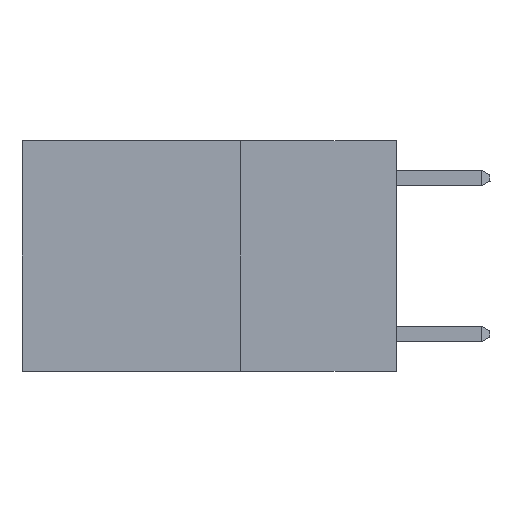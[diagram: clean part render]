
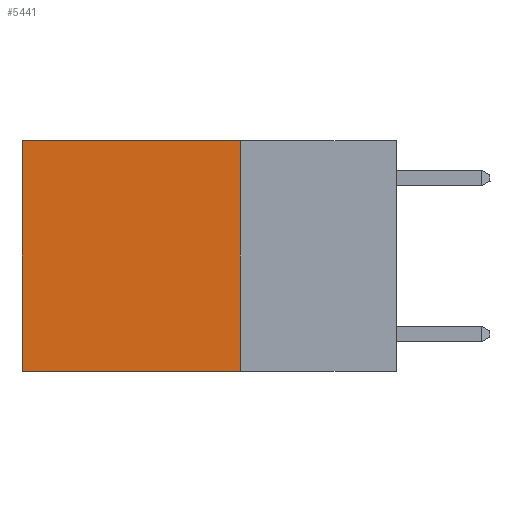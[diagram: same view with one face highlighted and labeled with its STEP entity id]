
A CAD part, left-side view. The second image highlights one B-rep face of the part: STEP entity #5441.
In plain terms, the highlighted planar face has unit normal (-1, 0, 0).
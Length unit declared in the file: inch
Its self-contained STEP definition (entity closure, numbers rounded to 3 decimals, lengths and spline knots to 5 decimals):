
#237 = CARTESIAN_POINT ( 'NONE',  ( 0.2625, 0.25, -0.37 ) ) ;
#318 = ORIENTED_EDGE ( 'NONE', *, *, #1720, .T. ) ;
#560 = ORIENTED_EDGE ( 'NONE', *, *, #9126, .T. ) ;
#706 = ORIENTED_EDGE ( 'NONE', *, *, #6501, .F. ) ;
#938 = VECTOR ( 'NONE', #12618, 39.37008 ) ;
#1126 = VERTEX_POINT ( 'NONE', #3888 ) ;
#1174 = VERTEX_POINT ( 'NONE', #10986 ) ;
#1469 = DIRECTION ( 'NONE',  ( 0., 1., 0. ) ) ;
#1720 = EDGE_CURVE ( 'NONE', #1126, #4855, #3247, .T. ) ;
#2049 = FACE_OUTER_BOUND ( 'NONE', #2755, .T. ) ;
#2755 = EDGE_LOOP ( 'NONE', ( #560, #706, #4745, #318 ) ) ;
#2825 = VECTOR ( 'NONE', #4161, 39.37008 ) ;
#3247 = LINE ( 'NONE', #10309, #15235 ) ;
#3888 = CARTESIAN_POINT ( 'NONE',  ( 0.2625, 0.25, 0. ) ) ;
#3931 = AXIS2_PLACEMENT_3D ( 'NONE', #5348, #4150, #12675 ) ;
#4082 = VERTEX_POINT ( 'NONE', #11583 ) ;
#4150 = DIRECTION ( 'NONE',  ( 1., 0., 0. ) ) ;
#4161 = DIRECTION ( 'NONE',  ( 0., 0., -1. ) ) ;
#4568 = LINE ( 'NONE', #5341, #938 ) ;
#4745 = ORIENTED_EDGE ( 'NONE', *, *, #9727, .F. ) ;
#4855 = VERTEX_POINT ( 'NONE', #8753 ) ;
#5341 = CARTESIAN_POINT ( 'NONE',  ( 0.2625, 0.25, 0. ) ) ;
#5348 = CARTESIAN_POINT ( 'NONE',  ( 0.2625, 0.25, 0. ) ) ;
#5441 = ADVANCED_FACE ( 'NONE', ( #2049 ), #9069, .F. ) ;
#6501 = EDGE_CURVE ( 'NONE', #1174, #4082, #13908, .T. ) ;
#8753 = CARTESIAN_POINT ( 'NONE',  ( 0.2625, 0.6, 0. ) ) ;
#9069 = PLANE ( 'NONE',  #3931 ) ;
#9126 = EDGE_CURVE ( 'NONE', #4855, #4082, #9400, .T. ) ;
#9400 = LINE ( 'NONE', #10271, #2825 ) ;
#9727 = EDGE_CURVE ( 'NONE', #1126, #1174, #4568, .T. ) ;
#10271 = CARTESIAN_POINT ( 'NONE',  ( 0.2625, 0.6, 0. ) ) ;
#10309 = CARTESIAN_POINT ( 'NONE',  ( 0.2625, 0.25, 0. ) ) ;
#10986 = CARTESIAN_POINT ( 'NONE',  ( 0.2625, 0.25, -0.37 ) ) ;
#11583 = CARTESIAN_POINT ( 'NONE',  ( 0.2625, 0.6, -0.37 ) ) ;
#12618 = DIRECTION ( 'NONE',  ( 0., 0., -1. ) ) ;
#12675 = DIRECTION ( 'NONE',  ( 0., 0., -1. ) ) ;
#13293 = DIRECTION ( 'NONE',  ( 0., 1., 0. ) ) ;
#13576 = VECTOR ( 'NONE', #1469, 39.37008 ) ;
#13908 = LINE ( 'NONE', #237, #13576 ) ;
#15235 = VECTOR ( 'NONE', #13293, 39.37008 ) ;
